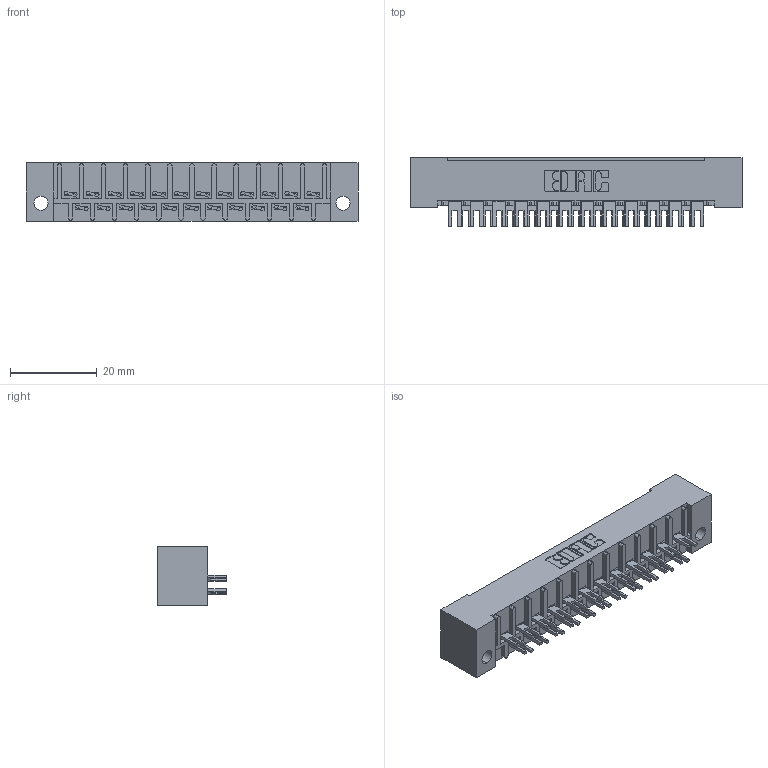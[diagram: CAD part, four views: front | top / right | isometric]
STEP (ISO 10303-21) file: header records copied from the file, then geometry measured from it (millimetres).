
FILE_DESCRIPTION (( 'STEP AP203' ), '1' );
FILE_NAME ('408-023-502-112.STEP', '2019-11-04T18:41:23', ( '' ), ( '' ), 'SwSTEP 2.0', 'SolidWorks 2016', '' );
FILE_SCHEMA (( 'CONFIG_CONTROL_DESIGN' ));
Length unit declared in the file: inch
Products named in the file (3): 408-023-502-112; 408 Part_023 - 1; 408-290-001_408-290-102
Assembly tree (24 placements, depth 2):
  408-023-502-112
    408 Part_023 - 1
    408-290-001_408-290-102  x23
Bounding box: 76.35 x 15.77 x 13.49 mm (x, y, z)
Volume: 8907 mm3; surface area: 10328.3 mm2
Topology: 24 solids, 24 shells, 1346 faces, 3688 edges, 2396 vertices
Faces by surface type: plane 1022, cylinder 232, bspline 92
Entity records: 19291 total; most frequent: CARTESIAN_POINT 3333, ORIENTED_EDGE 3240, DIRECTION 2966, EDGE_CURVE 1620, VECTOR 1420, LINE 1420, VERTEX_POINT 1076, AXIS2_PLACEMENT_3D 773
